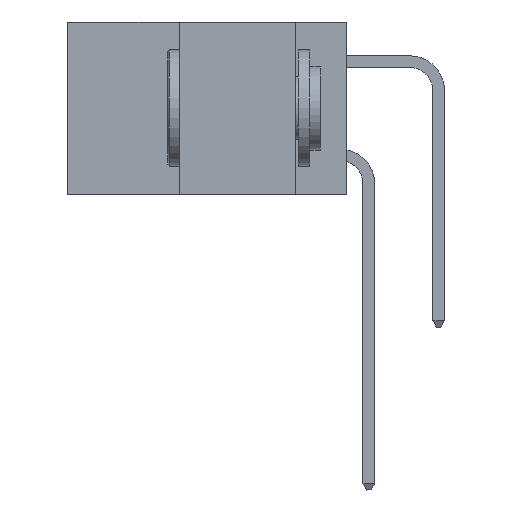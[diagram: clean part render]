
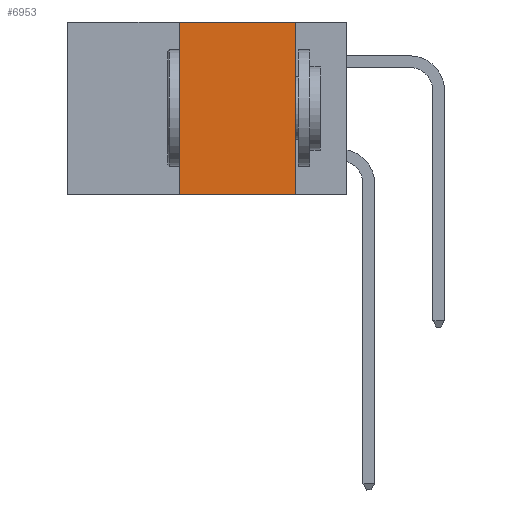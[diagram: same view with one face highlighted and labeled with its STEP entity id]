
A CAD part, left-side view. The second image highlights one B-rep face of the part: STEP entity #6953.
In plain terms, the highlighted planar face has unit normal (-1, 0, 0).
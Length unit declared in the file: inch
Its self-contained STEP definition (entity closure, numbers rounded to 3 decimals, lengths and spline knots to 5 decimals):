
#314 = CARTESIAN_POINT ( 'NONE',  ( 0., 0.36, 0. ) ) ;
#928 = DIRECTION ( 'NONE',  ( 0., 0., 1. ) ) ;
#2710 = VECTOR ( 'NONE', #19633, 39.37008 ) ;
#3814 = EDGE_CURVE ( 'NONE', #5215, #18633, #19398, .T. ) ;
#4130 = VERTEX_POINT ( 'NONE', #6179 ) ;
#4838 = LINE ( 'NONE', #9786, #2710 ) ;
#5215 = VERTEX_POINT ( 'NONE', #314 ) ;
#5227 = FACE_OUTER_BOUND ( 'NONE', #9649, .T. ) ;
#5266 = DIRECTION ( 'NONE',  ( 0., 0., -1. ) ) ;
#6179 = CARTESIAN_POINT ( 'NONE',  ( 0., 0.11, -0.37 ) ) ;
#6780 = VERTEX_POINT ( 'NONE', #23937 ) ;
#6953 = ADVANCED_FACE ( 'NONE', ( #5227 ), #20790, .F. ) ;
#7610 = VECTOR ( 'NONE', #928, 39.37008 ) ;
#8504 = LINE ( 'NONE', #10800, #7610 ) ;
#8639 = ORIENTED_EDGE ( 'NONE', *, *, #24856, .F. ) ;
#9050 = VECTOR ( 'NONE', #14371, 39.37008 ) ;
#9383 = LINE ( 'NONE', #12527, #9050 ) ;
#9420 = CARTESIAN_POINT ( 'NONE',  ( 0., 0.6, 0. ) ) ;
#9649 = EDGE_LOOP ( 'NONE', ( #24901, #13543, #8639, #19410 ) ) ;
#9786 = CARTESIAN_POINT ( 'NONE',  ( 0., 0.6, -0.37 ) ) ;
#10800 = CARTESIAN_POINT ( 'NONE',  ( 0., 0.36, 0. ) ) ;
#11406 = DIRECTION ( 'NONE',  ( 0., -1., 0. ) ) ;
#12272 = AXIS2_PLACEMENT_3D ( 'NONE', #22764, #18587, #5266 ) ;
#12485 = EDGE_CURVE ( 'NONE', #18633, #4130, #9383, .T. ) ;
#12527 = CARTESIAN_POINT ( 'NONE',  ( 0., 0.11, 0. ) ) ;
#13543 = ORIENTED_EDGE ( 'NONE', *, *, #3814, .F. ) ;
#13620 = VECTOR ( 'NONE', #11406, 39.37008 ) ;
#14371 = DIRECTION ( 'NONE',  ( 0., 0., -1. ) ) ;
#17562 = EDGE_CURVE ( 'NONE', #6780, #4130, #4838, .T. ) ;
#18587 = DIRECTION ( 'NONE',  ( 1., 0., 0. ) ) ;
#18633 = VERTEX_POINT ( 'NONE', #19103 ) ;
#19103 = CARTESIAN_POINT ( 'NONE',  ( 0., 0.11, 0. ) ) ;
#19398 = LINE ( 'NONE', #9420, #13620 ) ;
#19410 = ORIENTED_EDGE ( 'NONE', *, *, #17562, .T. ) ;
#19633 = DIRECTION ( 'NONE',  ( 0., -1., 0. ) ) ;
#20790 = PLANE ( 'NONE',  #12272 ) ;
#22764 = CARTESIAN_POINT ( 'NONE',  ( 0., 0.6, 0. ) ) ;
#23937 = CARTESIAN_POINT ( 'NONE',  ( 0., 0.36, -0.37 ) ) ;
#24856 = EDGE_CURVE ( 'NONE', #6780, #5215, #8504, .T. ) ;
#24901 = ORIENTED_EDGE ( 'NONE', *, *, #12485, .F. ) ;
